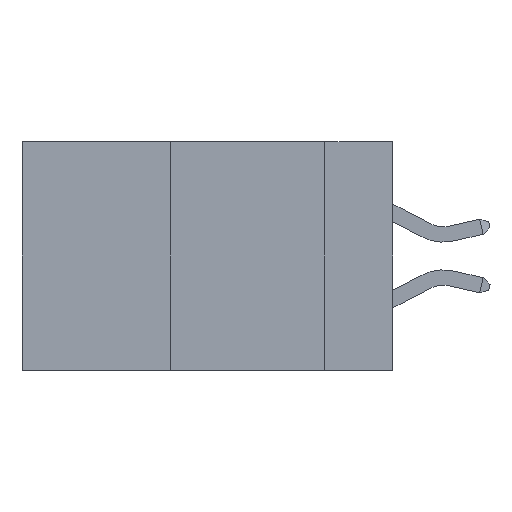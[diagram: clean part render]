
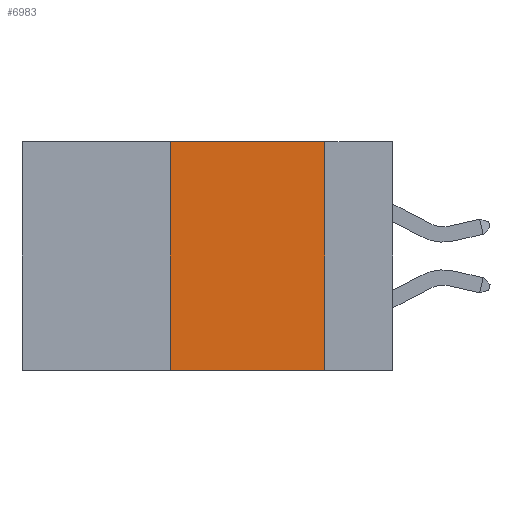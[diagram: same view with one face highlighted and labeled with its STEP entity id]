
A CAD part, left-side view. The second image highlights one B-rep face of the part: STEP entity #6983.
In plain terms, the highlighted planar face has unit normal (-1, 0, 0).
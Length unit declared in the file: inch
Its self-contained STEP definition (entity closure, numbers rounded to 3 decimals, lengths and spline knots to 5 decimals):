
#1173 = CARTESIAN_POINT ( 'NONE',  ( 0., 0.11, -0.37 ) ) ;
#1528 = EDGE_CURVE ( 'NONE', #8556, #8601, #5357, .T. ) ;
#1723 = ORIENTED_EDGE ( 'NONE', *, *, #13511, .F. ) ;
#2220 = CARTESIAN_POINT ( 'NONE',  ( 0., 0.36, 0. ) ) ;
#2310 = EDGE_CURVE ( 'NONE', #8556, #12648, #4037, .T. ) ;
#2993 = DIRECTION ( 'NONE',  ( 0., 0., -1. ) ) ;
#4037 = LINE ( 'NONE', #9360, #4413 ) ;
#4407 = LINE ( 'NONE', #4796, #4790 ) ;
#4413 = VECTOR ( 'NONE', #11156, 39.37008 ) ;
#4766 = VECTOR ( 'NONE', #12581, 39.37008 ) ;
#4790 = VECTOR ( 'NONE', #13407, 39.37008 ) ;
#4796 = CARTESIAN_POINT ( 'NONE',  ( 0., 0.6, 0. ) ) ;
#4830 = EDGE_LOOP ( 'NONE', ( #1723, #10976, #14464, #12161 ) ) ;
#5357 = LINE ( 'NONE', #2220, #13568 ) ;
#5422 = FACE_OUTER_BOUND ( 'NONE', #4830, .T. ) ;
#6714 = AXIS2_PLACEMENT_3D ( 'NONE', #8712, #9766, #2993 ) ;
#6983 = ADVANCED_FACE ( 'NONE', ( #5422 ), #11821, .F. ) ;
#7005 = CARTESIAN_POINT ( 'NONE',  ( 0., 0.36, 0. ) ) ;
#7249 = CARTESIAN_POINT ( 'NONE',  ( 0., 0.11, 0. ) ) ;
#8048 = DIRECTION ( 'NONE',  ( 0., 0., 1. ) ) ;
#8556 = VERTEX_POINT ( 'NONE', #14291 ) ;
#8601 = VERTEX_POINT ( 'NONE', #7005 ) ;
#8712 = CARTESIAN_POINT ( 'NONE',  ( 0., 0.6, 0. ) ) ;
#9360 = CARTESIAN_POINT ( 'NONE',  ( 0., 0.6, -0.37 ) ) ;
#9419 = VERTEX_POINT ( 'NONE', #10343 ) ;
#9766 = DIRECTION ( 'NONE',  ( 1., 0., 0. ) ) ;
#10343 = CARTESIAN_POINT ( 'NONE',  ( 0., 0.11, 0. ) ) ;
#10976 = ORIENTED_EDGE ( 'NONE', *, *, #12116, .F. ) ;
#11156 = DIRECTION ( 'NONE',  ( 0., -1., 0. ) ) ;
#11288 = LINE ( 'NONE', #7249, #4766 ) ;
#11821 = PLANE ( 'NONE',  #6714 ) ;
#12116 = EDGE_CURVE ( 'NONE', #8601, #9419, #4407, .T. ) ;
#12161 = ORIENTED_EDGE ( 'NONE', *, *, #2310, .T. ) ;
#12581 = DIRECTION ( 'NONE',  ( 0., 0., -1. ) ) ;
#12648 = VERTEX_POINT ( 'NONE', #1173 ) ;
#13407 = DIRECTION ( 'NONE',  ( 0., -1., 0. ) ) ;
#13511 = EDGE_CURVE ( 'NONE', #9419, #12648, #11288, .T. ) ;
#13568 = VECTOR ( 'NONE', #8048, 39.37008 ) ;
#14291 = CARTESIAN_POINT ( 'NONE',  ( 0., 0.36, -0.37 ) ) ;
#14464 = ORIENTED_EDGE ( 'NONE', *, *, #1528, .F. ) ;
